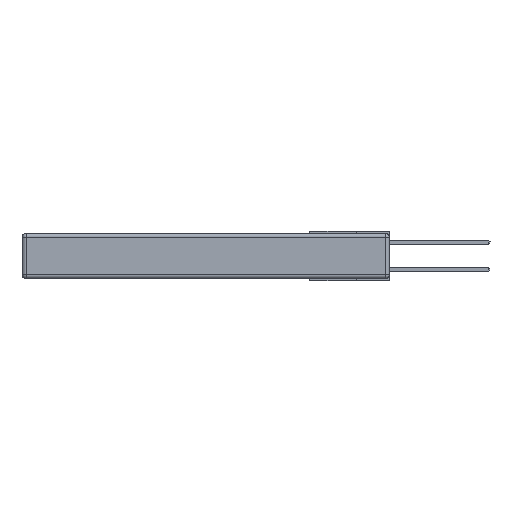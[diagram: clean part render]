
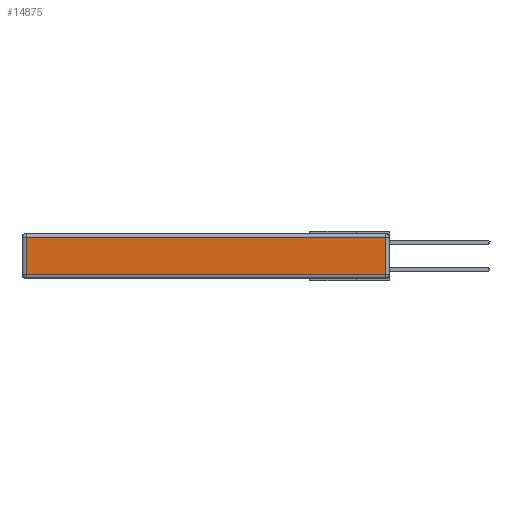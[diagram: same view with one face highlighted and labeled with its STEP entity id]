
A CAD part, left-side view. The second image highlights one B-rep face of the part: STEP entity #14875.
In plain terms, the highlighted planar face has unit normal (-1, 0, 0).
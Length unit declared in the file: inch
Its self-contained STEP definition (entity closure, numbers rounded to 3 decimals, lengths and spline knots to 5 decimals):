
#2139 = LINE ( 'NONE', #32159, #30601 ) ;
#2486 = ORIENTED_EDGE ( 'NONE', *, *, #30102, .T. ) ;
#2588 = DIRECTION ( 'NONE',  ( -1., 0., 0. ) ) ;
#2797 = LINE ( 'NONE', #3037, #26675 ) ;
#3037 = CARTESIAN_POINT ( 'NONE',  ( 0., 2.75, -0.03 ) ) ;
#3331 = DIRECTION ( 'NONE',  ( 0., 0., -1. ) ) ;
#4383 = VERTEX_POINT ( 'NONE', #21513 ) ;
#4488 = LINE ( 'NONE', #20921, #17200 ) ;
#7489 = DIRECTION ( 'NONE',  ( 0., 0., 1. ) ) ;
#12916 = EDGE_CURVE ( 'NONE', #30185, #26987, #2139, .T. ) ;
#14003 = CARTESIAN_POINT ( 'NONE',  ( 0., 0., -0.313 ) ) ;
#14538 = AXIS2_PLACEMENT_3D ( 'NONE', #33767, #2588, #16242 ) ;
#14875 = ADVANCED_FACE ( 'NONE', ( #21173 ), #32103, .T. ) ;
#16242 = DIRECTION ( 'NONE',  ( 0., 0., 1. ) ) ;
#17200 = VECTOR ( 'NONE', #7489, 39.37008 ) ;
#18117 = CARTESIAN_POINT ( 'NONE',  ( 0., 2.72, -0.03 ) ) ;
#19362 = ORIENTED_EDGE ( 'NONE', *, *, #12916, .T. ) ;
#20253 = CARTESIAN_POINT ( 'NONE',  ( 0., 0.03, -0.03 ) ) ;
#20921 = CARTESIAN_POINT ( 'NONE',  ( 0., 0.03, -0.343 ) ) ;
#21173 = FACE_OUTER_BOUND ( 'NONE', #22187, .T. ) ;
#21513 = CARTESIAN_POINT ( 'NONE',  ( 0., 0.03, -0.313 ) ) ;
#22187 = EDGE_LOOP ( 'NONE', ( #24526, #24990, #2486, #19362 ) ) ;
#23696 = VECTOR ( 'NONE', #27956, 39.37008 ) ;
#24526 = ORIENTED_EDGE ( 'NONE', *, *, #31369, .T. ) ;
#24990 = ORIENTED_EDGE ( 'NONE', *, *, #31691, .T. ) ;
#26675 = VECTOR ( 'NONE', #30289, 39.37008 ) ;
#26987 = VERTEX_POINT ( 'NONE', #32330 ) ;
#27956 = DIRECTION ( 'NONE',  ( 0., -1., 0. ) ) ;
#30102 = EDGE_CURVE ( 'NONE', #34945, #30185, #2797, .T. ) ;
#30185 = VERTEX_POINT ( 'NONE', #18117 ) ;
#30289 = DIRECTION ( 'NONE',  ( 0., 1., 0. ) ) ;
#30601 = VECTOR ( 'NONE', #3331, 39.37008 ) ;
#31369 = EDGE_CURVE ( 'NONE', #26987, #4383, #31380, .T. ) ;
#31380 = LINE ( 'NONE', #14003, #23696 ) ;
#31691 = EDGE_CURVE ( 'NONE', #4383, #34945, #4488, .T. ) ;
#32103 = PLANE ( 'NONE',  #14538 ) ;
#32159 = CARTESIAN_POINT ( 'NONE',  ( 0., 2.72, -0.343 ) ) ;
#32330 = CARTESIAN_POINT ( 'NONE',  ( 0., 2.72, -0.313 ) ) ;
#33767 = CARTESIAN_POINT ( 'NONE',  ( 0., 0., -0.343 ) ) ;
#34945 = VERTEX_POINT ( 'NONE', #20253 ) ;
